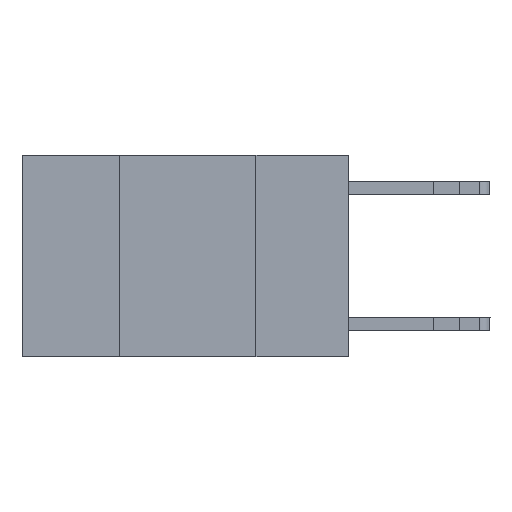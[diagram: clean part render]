
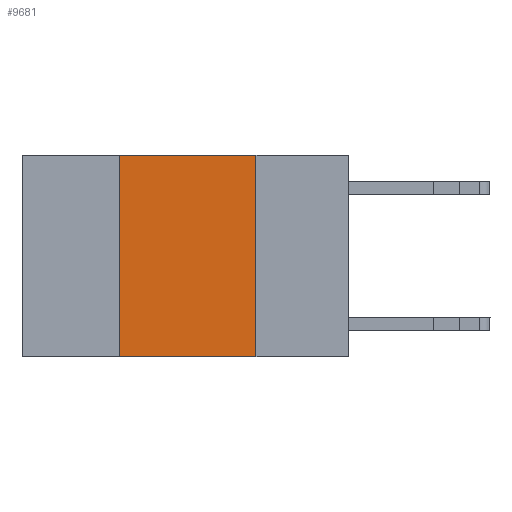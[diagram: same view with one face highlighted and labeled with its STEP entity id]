
A CAD part, left-side view. The second image highlights one B-rep face of the part: STEP entity #9681.
In plain terms, the highlighted planar face has unit normal (-1, 0, 0).
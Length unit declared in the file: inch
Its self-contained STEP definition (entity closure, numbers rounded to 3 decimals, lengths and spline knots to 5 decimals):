
#228 = CARTESIAN_POINT ( 'NONE',  ( 0., 0.42, -0.37 ) ) ;
#245 = VECTOR ( 'NONE', #2969, 39.37008 ) ;
#1329 = EDGE_LOOP ( 'NONE', ( #12294, #6518, #25462, #1739 ) ) ;
#1455 = AXIS2_PLACEMENT_3D ( 'NONE', #6255, #15011, #1975 ) ;
#1739 = ORIENTED_EDGE ( 'NONE', *, *, #21770, .T. ) ;
#1975 = DIRECTION ( 'NONE',  ( 0., 0., -1. ) ) ;
#2969 = DIRECTION ( 'NONE',  ( 0., 0., -1. ) ) ;
#3459 = DIRECTION ( 'NONE',  ( 0., -1., 0. ) ) ;
#4108 = LINE ( 'NONE', #26963, #25795 ) ;
#4687 = VERTEX_POINT ( 'NONE', #228 ) ;
#5154 = CARTESIAN_POINT ( 'NONE',  ( 0., 0.17, 0. ) ) ;
#5403 = DIRECTION ( 'NONE',  ( 0., -1., 0. ) ) ;
#6155 = VECTOR ( 'NONE', #3459, 39.37008 ) ;
#6255 = CARTESIAN_POINT ( 'NONE',  ( 0., 0.6, 0. ) ) ;
#6518 = ORIENTED_EDGE ( 'NONE', *, *, #9427, .F. ) ;
#9427 = EDGE_CURVE ( 'NONE', #26171, #17085, #4108, .T. ) ;
#9681 = ADVANCED_FACE ( 'NONE', ( #24110 ), #10623, .F. ) ;
#9974 = LINE ( 'NONE', #10274, #20773 ) ;
#10274 = CARTESIAN_POINT ( 'NONE',  ( 0., 0.42, 0. ) ) ;
#10586 = EDGE_CURVE ( 'NONE', #17085, #15381, #23309, .T. ) ;
#10623 = PLANE ( 'NONE',  #1455 ) ;
#12294 = ORIENTED_EDGE ( 'NONE', *, *, #10586, .F. ) ;
#12791 = EDGE_CURVE ( 'NONE', #4687, #26171, #9974, .T. ) ;
#14351 = CARTESIAN_POINT ( 'NONE',  ( 0., 0.17, -0.37 ) ) ;
#15011 = DIRECTION ( 'NONE',  ( 1., 0., 0. ) ) ;
#15381 = VERTEX_POINT ( 'NONE', #14351 ) ;
#17085 = VERTEX_POINT ( 'NONE', #24030 ) ;
#18347 = LINE ( 'NONE', #20888, #6155 ) ;
#18406 = CARTESIAN_POINT ( 'NONE',  ( 0., 0.42, 0. ) ) ;
#20773 = VECTOR ( 'NONE', #27457, 39.37008 ) ;
#20888 = CARTESIAN_POINT ( 'NONE',  ( 0., 0.6, -0.37 ) ) ;
#21770 = EDGE_CURVE ( 'NONE', #4687, #15381, #18347, .T. ) ;
#23309 = LINE ( 'NONE', #5154, #245 ) ;
#24030 = CARTESIAN_POINT ( 'NONE',  ( 0., 0.17, 0. ) ) ;
#24110 = FACE_OUTER_BOUND ( 'NONE', #1329, .T. ) ;
#25462 = ORIENTED_EDGE ( 'NONE', *, *, #12791, .F. ) ;
#25795 = VECTOR ( 'NONE', #5403, 39.37008 ) ;
#26171 = VERTEX_POINT ( 'NONE', #18406 ) ;
#26963 = CARTESIAN_POINT ( 'NONE',  ( 0., 0.6, 0. ) ) ;
#27457 = DIRECTION ( 'NONE',  ( 0., 0., 1. ) ) ;
